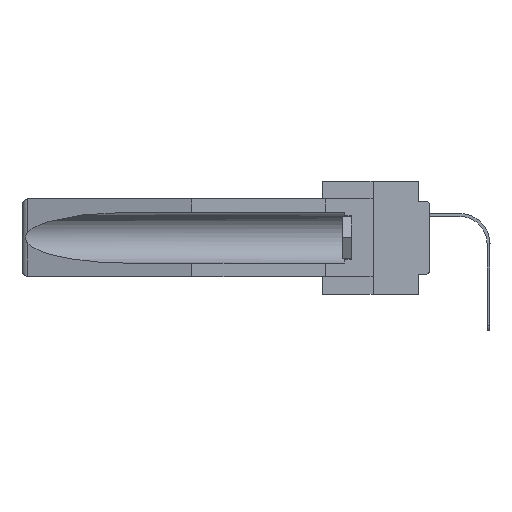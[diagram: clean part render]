
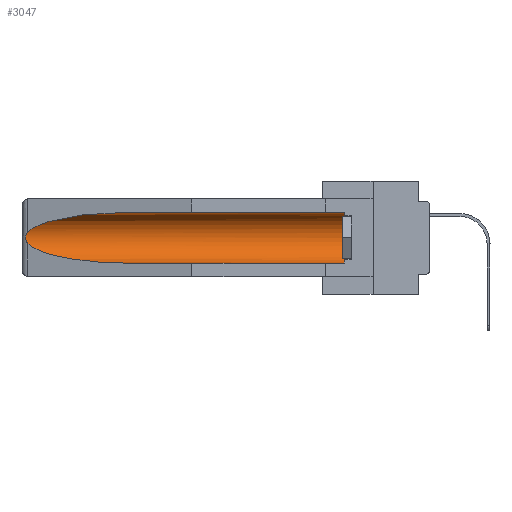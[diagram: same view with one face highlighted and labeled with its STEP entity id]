
A CAD part, left-side view. The second image highlights one B-rep face of the part: STEP entity #3047.
In plain terms, the highlighted cylindrical face has radius 2.857 mm (diameter 5.715 mm), a partial arc.
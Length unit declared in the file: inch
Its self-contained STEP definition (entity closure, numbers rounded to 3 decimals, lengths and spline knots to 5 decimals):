
#496 = DIRECTION ( 'NONE',  ( 0., 1., 0. ) ) ;
#625 = CARTESIAN_POINT ( 'NONE',  ( 0.2675, 1.53308, -0.16763 ) ) ;
#634 = CARTESIAN_POINT ( 'NONE',  ( 0.155, -0.30754, -0.284 ) ) ;
#756 = CARTESIAN_POINT ( 'NONE',  ( 0.25451, 1.48313, -0.24835 ) ) ;
#770 = CARTESIAN_POINT ( 'NONE',  ( 0.2675, 1.53308, -0.17534 ) ) ;
#841 = CARTESIAN_POINT ( 'NONE',  ( 0.155, 1.07973, -0.059 ) ) ;
#1401 = CARTESIAN_POINT ( 'NONE',  ( 0.26537, 1.52718, -0.14972 ) ) ;
#1866 = CARTESIAN_POINT ( 'NONE',  ( 0.155, 0.126, -0.284 ) ) ;
#2176 = CARTESIAN_POINT ( 'NONE',  ( 0.26537, 1.52718, -0.19328 ) ) ;
#2178 = VERTEX_POINT ( 'NONE', #18632 ) ;
#3047 = ADVANCED_FACE ( 'NONE', ( #9175 ), #14031, .F. ) ;
#3224 = DIRECTION ( 'NONE',  ( 0., -1., 0. ) ) ;
#3269 = DIRECTION ( 'NONE',  ( 0., 1., 0. ) ) ;
#5317 = CARTESIAN_POINT ( 'NONE',  ( 0.2673, 1.53269, -0.17917 ) ) ;
#6541 = VECTOR ( 'NONE', #3269, 39.37008 ) ;
#6992 = CIRCLE ( 'NONE', #15462, 0.1125 ) ;
#7034 = CARTESIAN_POINT ( 'NONE',  ( 0.155, 1.07973, -0.284 ) ) ;
#7532 = CARTESIAN_POINT ( 'NONE',  ( 0.26597, 1.52961, -0.15275 ) ) ;
#7921 = CARTESIAN_POINT ( 'NONE',  ( 0.155, 0.126, -0.1715 ) ) ;
#8295 =( BOUNDED_CURVE ( )  B_SPLINE_CURVE ( 3, ( #841, #11864, #25371, #16584 ),
 .UNSPECIFIED., .F., .T. ) 
 B_SPLINE_CURVE_WITH_KNOTS ( ( 4, 4 ),
 ( 4.71239, 6.08839 ),
 .UNSPECIFIED. ) 
 CURVE ( )  GEOMETRIC_REPRESENTATION_ITEM ( )  RATIONAL_B_SPLINE_CURVE ( ( 1., 0.848, 0.848, 1. ) ) 
 REPRESENTATION_ITEM ( '' )  );
#8345 = CARTESIAN_POINT ( 'NONE',  ( 0.155, 1.07973, -0.284 ) ) ;
#8405 = EDGE_CURVE ( 'NONE', #27906, #24281, #19542, .T. ) ;
#9175 = FACE_OUTER_BOUND ( 'NONE', #17251, .T. ) ;
#10034 = B_SPLINE_CURVE_WITH_KNOTS ( 'NONE', 3,
 ( #20910, #7532, #20768, #11933, #625, #770, #5317, #14300, #16515, #18697 ),
 .UNSPECIFIED., .F., .F.,
 ( 4, 2, 2, 2, 4 ),
 ( 0., 0.00029, 0.00058, 0.00087, 0.00117 ),
 .UNSPECIFIED. ) ;
#10873 = CARTESIAN_POINT ( 'NONE',  ( 0.21114, 1.30732, -0.284 ) ) ;
#11864 = CARTESIAN_POINT ( 'NONE',  ( 0.21114, 1.30732, -0.059 ) ) ;
#11876 = EDGE_CURVE ( 'NONE', #24298, #24281, #18857, .T. ) ;
#11933 = CARTESIAN_POINT ( 'NONE',  ( 0.2673, 1.5327, -0.16383 ) ) ;
#13133 = ORIENTED_EDGE ( 'NONE', *, *, #21495, .T. ) ;
#13887 = CARTESIAN_POINT ( 'NONE',  ( 0.155, -0.30754, -0.1715 ) ) ;
#14031 = CYLINDRICAL_SURFACE ( 'NONE', #27335, 0.1125 ) ;
#14300 = CARTESIAN_POINT ( 'NONE',  ( 0.26655, 1.53094, -0.18657 ) ) ;
#14332 = DIRECTION ( 'NONE',  ( 0., 1., 0. ) ) ;
#15074 = VECTOR ( 'NONE', #14332, 39.37008 ) ;
#15462 = AXIS2_PLACEMENT_3D ( 'NONE', #7921, #3224, #16907 ) ;
#15634 = CARTESIAN_POINT ( 'NONE',  ( 0.26537, 1.52718, -0.19328 ) ) ;
#16351 = ORIENTED_EDGE ( 'NONE', *, *, #8405, .T. ) ;
#16515 = CARTESIAN_POINT ( 'NONE',  ( 0.26597, 1.5296, -0.19026 ) ) ;
#16584 = CARTESIAN_POINT ( 'NONE',  ( 0.26537, 1.52718, -0.14972 ) ) ;
#16907 = DIRECTION ( 'NONE',  ( 0., 0., 1. ) ) ;
#17251 = EDGE_LOOP ( 'NONE', ( #19443, #19850, #16351, #24110, #13133, #24131 ) ) ;
#17824 = EDGE_CURVE ( 'NONE', #2178, #24796, #8295, .T. ) ;
#18632 = CARTESIAN_POINT ( 'NONE',  ( 0.155, 1.07973, -0.059 ) ) ;
#18697 = CARTESIAN_POINT ( 'NONE',  ( 0.26537, 1.52718, -0.19328 ) ) ;
#18843 = VERTEX_POINT ( 'NONE', #21883 ) ;
#18857 = LINE ( 'NONE', #634, #6541 ) ;
#19018 = LINE ( 'NONE', #27980, #15074 ) ;
#19443 = ORIENTED_EDGE ( 'NONE', *, *, #17824, .T. ) ;
#19542 =( BOUNDED_CURVE ( )  B_SPLINE_CURVE ( 3, ( #2176, #756, #10873, #7034 ),
 .UNSPECIFIED., .F., .F. ) 
 B_SPLINE_CURVE_WITH_KNOTS ( ( 4, 4 ),
 ( 0.1948, 1.5708 ),
 .UNSPECIFIED. ) 
 CURVE ( )  GEOMETRIC_REPRESENTATION_ITEM ( )  RATIONAL_B_SPLINE_CURVE ( ( 1., 0.848, 0.848, 1. ) ) 
 REPRESENTATION_ITEM ( '' )  );
#19850 = ORIENTED_EDGE ( 'NONE', *, *, #28031, .T. ) ;
#20768 = CARTESIAN_POINT ( 'NONE',  ( 0.26654, 1.53092, -0.15636 ) ) ;
#20910 = CARTESIAN_POINT ( 'NONE',  ( 0.26537, 1.52718, -0.14972 ) ) ;
#21495 = EDGE_CURVE ( 'NONE', #24298, #18843, #6992, .T. ) ;
#21883 = CARTESIAN_POINT ( 'NONE',  ( 0.155, 0.126, -0.059 ) ) ;
#22977 = DIRECTION ( 'NONE',  ( 0., 0., 1. ) ) ;
#24110 = ORIENTED_EDGE ( 'NONE', *, *, #11876, .F. ) ;
#24131 = ORIENTED_EDGE ( 'NONE', *, *, #27647, .T. ) ;
#24281 = VERTEX_POINT ( 'NONE', #8345 ) ;
#24298 = VERTEX_POINT ( 'NONE', #1866 ) ;
#24796 = VERTEX_POINT ( 'NONE', #1401 ) ;
#25371 = CARTESIAN_POINT ( 'NONE',  ( 0.25451, 1.48313, -0.09465 ) ) ;
#27335 = AXIS2_PLACEMENT_3D ( 'NONE', #13887, #496, #22977 ) ;
#27647 = EDGE_CURVE ( 'NONE', #18843, #2178, #19018, .T. ) ;
#27906 = VERTEX_POINT ( 'NONE', #15634 ) ;
#27980 = CARTESIAN_POINT ( 'NONE',  ( 0.155, -0.30754, -0.059 ) ) ;
#28031 = EDGE_CURVE ( 'NONE', #24796, #27906, #10034, .T. ) ;
